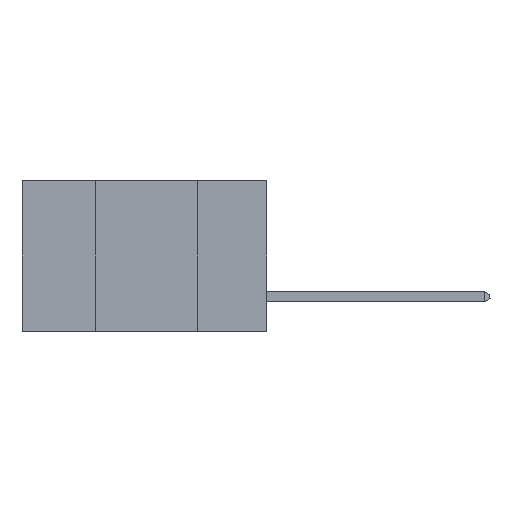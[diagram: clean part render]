
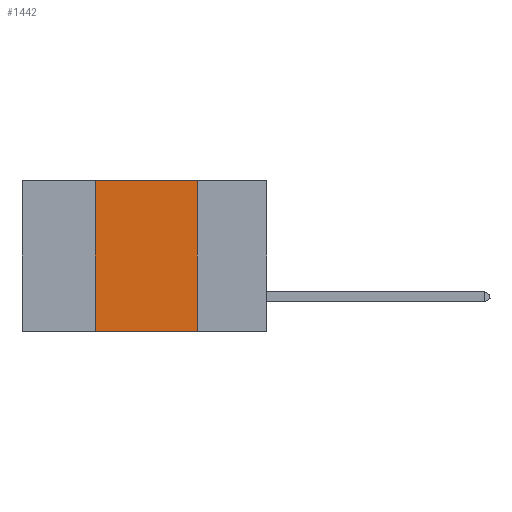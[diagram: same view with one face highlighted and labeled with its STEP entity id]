
A CAD part, left-side view. The second image highlights one B-rep face of the part: STEP entity #1442.
In plain terms, the highlighted planar face has unit normal (-1, 0, 0).
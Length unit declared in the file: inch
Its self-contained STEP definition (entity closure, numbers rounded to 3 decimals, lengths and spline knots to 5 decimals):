
#724 = EDGE_CURVE ( 'NONE', #18195, #6744, #13623, .T. ) ;
#1017 = DIRECTION ( 'NONE',  ( 0., -1., 0. ) ) ;
#1211 = CARTESIAN_POINT ( 'NONE',  ( 0., 0.17, -0.37 ) ) ;
#1442 = ADVANCED_FACE ( 'NONE', ( #18589 ), #3811, .F. ) ;
#2983 = LINE ( 'NONE', #16514, #15502 ) ;
#3000 = CARTESIAN_POINT ( 'NONE',  ( 0., 0.42, 0. ) ) ;
#3414 = EDGE_CURVE ( 'NONE', #9915, #7175, #21050, .T. ) ;
#3486 = ORIENTED_EDGE ( 'NONE', *, *, #724, .T. ) ;
#3533 = AXIS2_PLACEMENT_3D ( 'NONE', #10576, #12379, #14700 ) ;
#3811 = PLANE ( 'NONE',  #3533 ) ;
#4056 = CARTESIAN_POINT ( 'NONE',  ( 0., 0.17, 0. ) ) ;
#5505 = DIRECTION ( 'NONE',  ( 0., -1., 0. ) ) ;
#6744 = VERTEX_POINT ( 'NONE', #1211 ) ;
#7175 = VERTEX_POINT ( 'NONE', #4056 ) ;
#8417 = LINE ( 'NONE', #22281, #16194 ) ;
#8538 = VECTOR ( 'NONE', #5505, 39.37008 ) ;
#8586 = EDGE_CURVE ( 'NONE', #18195, #9915, #2983, .T. ) ;
#9329 = DIRECTION ( 'NONE',  ( 0., 0., 1. ) ) ;
#9703 = ORIENTED_EDGE ( 'NONE', *, *, #19707, .F. ) ;
#9915 = VERTEX_POINT ( 'NONE', #3000 ) ;
#10576 = CARTESIAN_POINT ( 'NONE',  ( 0., 0.6, 0. ) ) ;
#10631 = CARTESIAN_POINT ( 'NONE',  ( 0., 0.6, 0. ) ) ;
#11977 = CARTESIAN_POINT ( 'NONE',  ( 0., 0.42, -0.37 ) ) ;
#12379 = DIRECTION ( 'NONE',  ( 1., 0., 0. ) ) ;
#13623 = LINE ( 'NONE', #22117, #17513 ) ;
#14653 = EDGE_LOOP ( 'NONE', ( #9703, #16523, #17015, #3486 ) ) ;
#14700 = DIRECTION ( 'NONE',  ( 0., 0., -1. ) ) ;
#15502 = VECTOR ( 'NONE', #9329, 39.37008 ) ;
#16194 = VECTOR ( 'NONE', #20339, 39.37008 ) ;
#16514 = CARTESIAN_POINT ( 'NONE',  ( 0., 0.42, 0. ) ) ;
#16523 = ORIENTED_EDGE ( 'NONE', *, *, #3414, .F. ) ;
#17015 = ORIENTED_EDGE ( 'NONE', *, *, #8586, .F. ) ;
#17513 = VECTOR ( 'NONE', #1017, 39.37008 ) ;
#18195 = VERTEX_POINT ( 'NONE', #11977 ) ;
#18589 = FACE_OUTER_BOUND ( 'NONE', #14653, .T. ) ;
#19707 = EDGE_CURVE ( 'NONE', #7175, #6744, #8417, .T. ) ;
#20339 = DIRECTION ( 'NONE',  ( 0., 0., -1. ) ) ;
#21050 = LINE ( 'NONE', #10631, #8538 ) ;
#22117 = CARTESIAN_POINT ( 'NONE',  ( 0., 0.6, -0.37 ) ) ;
#22281 = CARTESIAN_POINT ( 'NONE',  ( 0., 0.17, 0. ) ) ;
